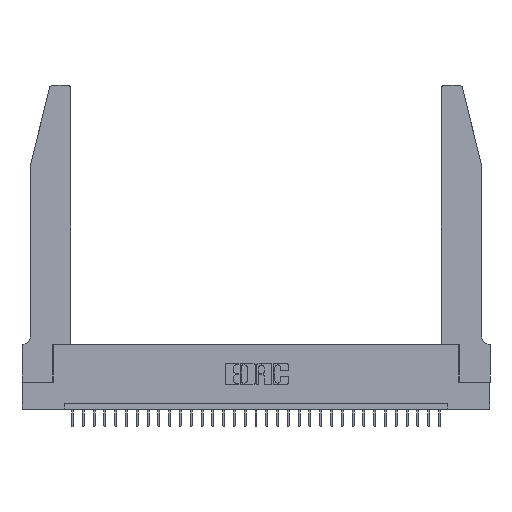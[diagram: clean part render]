
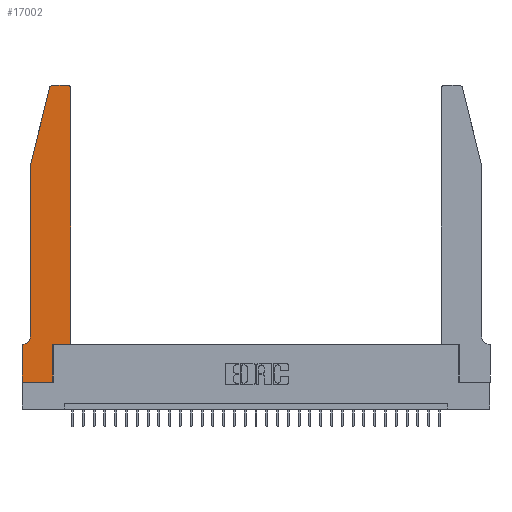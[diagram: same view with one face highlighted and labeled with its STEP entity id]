
A CAD part, top view. The second image highlights one B-rep face of the part: STEP entity #17002.
In plain terms, the highlighted planar face has unit normal (0, 0, 1).
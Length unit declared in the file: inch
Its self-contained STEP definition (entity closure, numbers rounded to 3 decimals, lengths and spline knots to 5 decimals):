
#559 = VERTEX_POINT ( 'NONE', #7971 ) ;
#601 = CARTESIAN_POINT ( 'NONE',  ( 0.284, 2.75, 0.37 ) ) ;
#700 = EDGE_CURVE ( 'NONE', #13340, #2193, #21391, .T. ) ;
#1147 = DIRECTION ( 'NONE',  ( -0.239, -0.971, 0. ) ) ;
#1191 = CARTESIAN_POINT ( 'NONE',  ( 0.4505, 0.35, 0.37 ) ) ;
#1715 = LINE ( 'NONE', #4261, #23130 ) ;
#2193 = VERTEX_POINT ( 'NONE', #23411 ) ;
#2251 = ORIENTED_EDGE ( 'NONE', *, *, #14621, .T. ) ;
#2776 = DIRECTION ( 'NONE',  ( 0., 0., 1. ) ) ;
#2883 = PLANE ( 'NONE',  #16266 ) ;
#3237 = CARTESIAN_POINT ( 'NONE',  ( 0.2865, 0., 0.37 ) ) ;
#3283 = ORIENTED_EDGE ( 'NONE', *, *, #21808, .T. ) ;
#3391 = EDGE_CURVE ( 'NONE', #559, #29425, #10990, .T. ) ;
#3946 = VECTOR ( 'NONE', #15900, 39.37008 ) ;
#4099 = CARTESIAN_POINT ( 'NONE',  ( 0.0755, 2., 0.37 ) ) ;
#4160 = EDGE_CURVE ( 'NONE', #23399, #23807, #8043, .T. ) ;
#4261 = CARTESIAN_POINT ( 'NONE',  ( 0.2865, 0.35, 0.37 ) ) ;
#4262 = DIRECTION ( 'NONE',  ( 1., 0., 0. ) ) ;
#5324 = ORIENTED_EDGE ( 'NONE', *, *, #14726, .T. ) ;
#5836 = LINE ( 'NONE', #1191, #11640 ) ;
#6405 = DIRECTION ( 'NONE',  ( 1., 0., 0. ) ) ;
#7686 = LINE ( 'NONE', #18613, #8837 ) ;
#7729 = VECTOR ( 'NONE', #31681, 39.37008 ) ;
#7895 = DIRECTION ( 'NONE',  ( -1., 0., 0. ) ) ;
#7971 = CARTESIAN_POINT ( 'NONE',  ( 0., 0., 0.37 ) ) ;
#8043 = LINE ( 'NONE', #18517, #13829 ) ;
#8213 = VECTOR ( 'NONE', #13992, 39.37008 ) ;
#8837 = VECTOR ( 'NONE', #1147, 39.37008 ) ;
#9017 = AXIS2_PLACEMENT_3D ( 'NONE', #9586, #13284, #29074 ) ;
#9284 = CARTESIAN_POINT ( 'NONE',  ( 0.4505, 0.35, 0.37 ) ) ;
#9586 = CARTESIAN_POINT ( 'NONE',  ( 0.284, 2.72, 0.37 ) ) ;
#10918 = EDGE_CURVE ( 'NONE', #2193, #14729, #28413, .T. ) ;
#10990 = LINE ( 'NONE', #18754, #27993 ) ;
#11009 = ORIENTED_EDGE ( 'NONE', *, *, #10918, .T. ) ;
#11135 = CARTESIAN_POINT ( 'NONE',  ( 0., 0., 0.37 ) ) ;
#11640 = VECTOR ( 'NONE', #21484, 39.37008 ) ;
#11891 = DIRECTION ( 'NONE',  ( 0., 0., 1. ) ) ;
#12098 = ORIENTED_EDGE ( 'NONE', *, *, #3391, .T. ) ;
#12850 = ORIENTED_EDGE ( 'NONE', *, *, #4160, .T. ) ;
#13284 = DIRECTION ( 'NONE',  ( 0., 0., 1. ) ) ;
#13340 = VERTEX_POINT ( 'NONE', #18781 ) ;
#13661 = AXIS2_PLACEMENT_3D ( 'NONE', #25169, #24958, #15209 ) ;
#13829 = VECTOR ( 'NONE', #23434, 39.37008 ) ;
#13992 = DIRECTION ( 'NONE',  ( 0., -1., 0. ) ) ;
#14359 = CARTESIAN_POINT ( 'NONE',  ( 0.0755, 0.35, 0.37 ) ) ;
#14569 = LINE ( 'NONE', #22880, #31625 ) ;
#14621 = EDGE_CURVE ( 'NONE', #21912, #13340, #7686, .T. ) ;
#14714 = LINE ( 'NONE', #14359, #7729 ) ;
#14726 = EDGE_CURVE ( 'NONE', #27951, #15393, #32102, .T. ) ;
#14729 = VERTEX_POINT ( 'NONE', #16125 ) ;
#15062 = ORIENTED_EDGE ( 'NONE', *, *, #31507, .T. ) ;
#15209 = DIRECTION ( 'NONE',  ( -1., 0., 0. ) ) ;
#15393 = VERTEX_POINT ( 'NONE', #17340 ) ;
#15900 = DIRECTION ( 'NONE',  ( 0., -1., 0. ) ) ;
#16125 = CARTESIAN_POINT ( 'NONE',  ( 0.0055, 0.35, 0.37 ) ) ;
#16266 = AXIS2_PLACEMENT_3D ( 'NONE', #20333, #2776, #18055 ) ;
#16499 = VERTEX_POINT ( 'NONE', #601 ) ;
#17002 = ADVANCED_FACE ( 'NONE', ( #17935 ), #2883, .T. ) ;
#17340 = CARTESIAN_POINT ( 'NONE',  ( 0.4205, 2.75, 0.37 ) ) ;
#17401 = ORIENTED_EDGE ( 'NONE', *, *, #17768, .T. ) ;
#17504 = EDGE_CURVE ( 'NONE', #16499, #21912, #30712, .T. ) ;
#17768 = EDGE_CURVE ( 'NONE', #19861, #559, #25314, .T. ) ;
#17935 = FACE_OUTER_BOUND ( 'NONE', #19992, .T. ) ;
#18055 = DIRECTION ( 'NONE',  ( 1., 0., 0. ) ) ;
#18517 = CARTESIAN_POINT ( 'NONE',  ( 0.4505, 0.35, 0.37 ) ) ;
#18613 = CARTESIAN_POINT ( 'NONE',  ( 0.0755, 2., 0.37 ) ) ;
#18754 = CARTESIAN_POINT ( 'NONE',  ( 0., 0., 0.37 ) ) ;
#18781 = CARTESIAN_POINT ( 'NONE',  ( 0.0755, 2., 0.37 ) ) ;
#19036 = DIRECTION ( 'NONE',  ( 0., 1., 0. ) ) ;
#19301 = CARTESIAN_POINT ( 'NONE',  ( 0.25487, 2.72718, 0.37 ) ) ;
#19360 = CARTESIAN_POINT ( 'NONE',  ( 0.4205, 2.72, 0.37 ) ) ;
#19861 = VERTEX_POINT ( 'NONE', #26610 ) ;
#19992 = EDGE_LOOP ( 'NONE', ( #20946, #26367, #2251, #28050, #11009, #15062, #17401, #12098, #23234, #12850, #3283, #5324 ) ) ;
#20333 = CARTESIAN_POINT ( 'NONE',  ( 0., 0.35, 0.37 ) ) ;
#20596 = CARTESIAN_POINT ( 'NONE',  ( 0.2865, 0.35, 0.37 ) ) ;
#20946 = ORIENTED_EDGE ( 'NONE', *, *, #26873, .T. ) ;
#21391 = LINE ( 'NONE', #4099, #8213 ) ;
#21484 = DIRECTION ( 'NONE',  ( 0., 1., 0. ) ) ;
#21808 = EDGE_CURVE ( 'NONE', #23807, #27951, #5836, .T. ) ;
#21912 = VERTEX_POINT ( 'NONE', #19301 ) ;
#22598 = CARTESIAN_POINT ( 'NONE',  ( 0.4505, 2.72, 0.37 ) ) ;
#22880 = CARTESIAN_POINT ( 'NONE',  ( 0.2605, 2.75, 0.37 ) ) ;
#23130 = VECTOR ( 'NONE', #19036, 39.37008 ) ;
#23234 = ORIENTED_EDGE ( 'NONE', *, *, #25519, .T. ) ;
#23399 = VERTEX_POINT ( 'NONE', #20596 ) ;
#23411 = CARTESIAN_POINT ( 'NONE',  ( 0.0755, 0.42, 0.37 ) ) ;
#23434 = DIRECTION ( 'NONE',  ( 1., 0., 0. ) ) ;
#23807 = VERTEX_POINT ( 'NONE', #9284 ) ;
#24536 = AXIS2_PLACEMENT_3D ( 'NONE', #19360, #11891, #4262 ) ;
#24958 = DIRECTION ( 'NONE',  ( 0., 0., -1. ) ) ;
#25169 = CARTESIAN_POINT ( 'NONE',  ( 0.0055, 0.42, 0.37 ) ) ;
#25314 = LINE ( 'NONE', #11135, #3946 ) ;
#25519 = EDGE_CURVE ( 'NONE', #29425, #23399, #1715, .T. ) ;
#26367 = ORIENTED_EDGE ( 'NONE', *, *, #17504, .T. ) ;
#26610 = CARTESIAN_POINT ( 'NONE',  ( 0., 0.35, 0.37 ) ) ;
#26873 = EDGE_CURVE ( 'NONE', #15393, #16499, #14569, .T. ) ;
#27951 = VERTEX_POINT ( 'NONE', #22598 ) ;
#27993 = VECTOR ( 'NONE', #6405, 39.37008 ) ;
#28050 = ORIENTED_EDGE ( 'NONE', *, *, #700, .T. ) ;
#28413 = CIRCLE ( 'NONE', #13661, 0.07 ) ;
#29074 = DIRECTION ( 'NONE',  ( 1., 0., 0. ) ) ;
#29425 = VERTEX_POINT ( 'NONE', #3237 ) ;
#30712 = CIRCLE ( 'NONE', #9017, 0.03 ) ;
#31507 = EDGE_CURVE ( 'NONE', #14729, #19861, #14714, .T. ) ;
#31625 = VECTOR ( 'NONE', #7895, 39.37008 ) ;
#31681 = DIRECTION ( 'NONE',  ( -1., 0., 0. ) ) ;
#32102 = CIRCLE ( 'NONE', #24536, 0.03 ) ;
